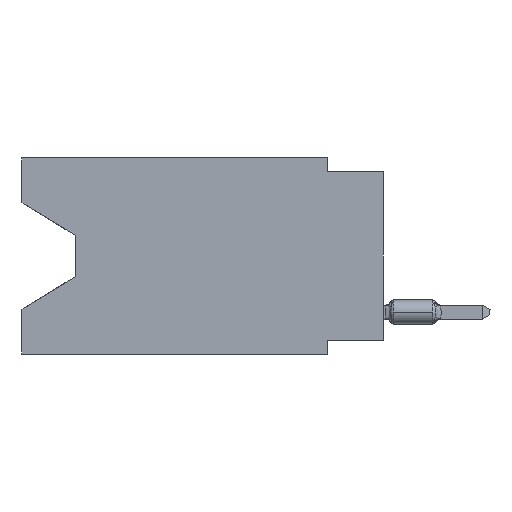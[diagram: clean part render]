
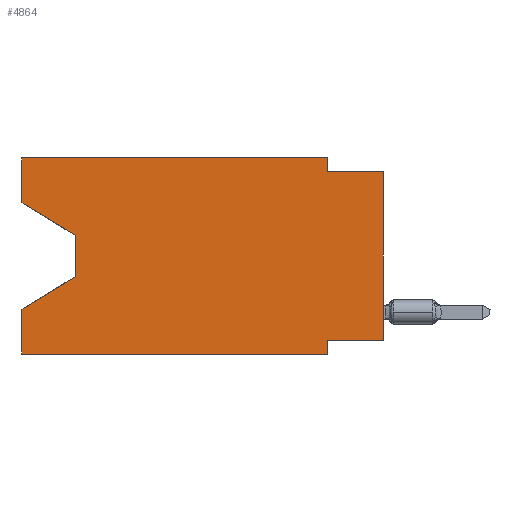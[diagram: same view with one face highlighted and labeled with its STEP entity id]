
A CAD part, left-side view. The second image highlights one B-rep face of the part: STEP entity #4864.
In plain terms, the highlighted planar face has unit normal (-1, 0, 0).
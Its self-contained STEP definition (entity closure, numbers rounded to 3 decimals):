
#112 = DIRECTION ( 'NONE',  ( 1., 0., 0. ) ) ;
#1184 = CARTESIAN_POINT ( 'NONE',  ( 0., 13.97, -5.385 ) ) ;
#3858 = VECTOR ( 'NONE', #36451, 1000. ) ;
#3903 = ORIENTED_EDGE ( 'NONE', *, *, #34705, .T. ) ;
#4229 = DIRECTION ( 'NONE',  ( 0., 1., 0. ) ) ;
#4771 = CARTESIAN_POINT ( 'NONE',  ( 0., 16.383, -6.852 ) ) ;
#4864 = ADVANCED_FACE ( 'NONE', ( #32024 ), #39775, .F. ) ;
#5009 = CARTESIAN_POINT ( 'NONE',  ( 0., 0., 0. ) ) ;
#5149 = CARTESIAN_POINT ( 'NONE',  ( 0., 2.54, 0. ) ) ;
#5249 = CARTESIAN_POINT ( 'NONE',  ( 0., 0., -8.255 ) ) ;
#6191 = DIRECTION ( 'NONE',  ( 0., 0., -1. ) ) ;
#6327 = VECTOR ( 'NONE', #29267, 1000. ) ;
#6953 = EDGE_CURVE ( 'NONE', #31298, #35868, #34721, .T. ) ;
#8057 = ORIENTED_EDGE ( 'NONE', *, *, #14320, .F. ) ;
#8295 = EDGE_CURVE ( 'NONE', #34327, #38568, #25600, .T. ) ;
#8542 = VERTEX_POINT ( 'NONE', #24056 ) ;
#9155 = EDGE_CURVE ( 'NONE', #8542, #35868, #26430, .T. ) ;
#9399 = DIRECTION ( 'NONE',  ( 0., -1., 0. ) ) ;
#9785 = DIRECTION ( 'NONE',  ( 0., 0., -1. ) ) ;
#9945 = DIRECTION ( 'NONE',  ( 0., -1., 0. ) ) ;
#10219 = ORIENTED_EDGE ( 'NONE', *, *, #41507, .T. ) ;
#10590 = CARTESIAN_POINT ( 'NONE',  ( 0., 2.54, -8.89 ) ) ;
#11214 = ORIENTED_EDGE ( 'NONE', *, *, #15917, .F. ) ;
#11377 = CARTESIAN_POINT ( 'NONE',  ( 0., 2.54, -8.255 ) ) ;
#12297 = EDGE_CURVE ( 'NONE', #21280, #42012, #35748, .T. ) ;
#12346 = VERTEX_POINT ( 'NONE', #10590 ) ;
#13457 = VERTEX_POINT ( 'NONE', #27858 ) ;
#13536 = CARTESIAN_POINT ( 'NONE',  ( 0., 0., -8.255 ) ) ;
#13543 = VERTEX_POINT ( 'NONE', #11377 ) ;
#13743 = DIRECTION ( 'NONE',  ( 0., 0.855, -0.519 ) ) ;
#14320 = EDGE_CURVE ( 'NONE', #37477, #8542, #21631, .T. ) ;
#14383 = CARTESIAN_POINT ( 'NONE',  ( 0., 13.97, -5.385 ) ) ;
#14740 = VECTOR ( 'NONE', #22101, 1000. ) ;
#14862 = EDGE_LOOP ( 'NONE', ( #21811, #34462, #3903, #35854, #10219, #37282, #26364, #19330, #38354, #8057, #11214, #35345 ) ) ;
#15600 = VECTOR ( 'NONE', #13743, 1000. ) ;
#15917 = EDGE_CURVE ( 'NONE', #13457, #37477, #33470, .T. ) ;
#16154 = CARTESIAN_POINT ( 'NONE',  ( 0., 16.383, 0. ) ) ;
#16544 = VECTOR ( 'NONE', #32602, 1000. ) ;
#16679 = CARTESIAN_POINT ( 'NONE',  ( 0., 0., -0.635 ) ) ;
#18980 = CARTESIAN_POINT ( 'NONE',  ( 0., 13.97, -3.505 ) ) ;
#18991 = VECTOR ( 'NONE', #9399, 1000. ) ;
#19330 = ORIENTED_EDGE ( 'NONE', *, *, #6953, .T. ) ;
#19361 = LINE ( 'NONE', #26292, #16544 ) ;
#19982 = CARTESIAN_POINT ( 'NONE',  ( 0., 2.54, 0. ) ) ;
#21280 = VERTEX_POINT ( 'NONE', #22576 ) ;
#21631 = LINE ( 'NONE', #5149, #28714 ) ;
#21811 = ORIENTED_EDGE ( 'NONE', *, *, #8295, .T. ) ;
#22101 = DIRECTION ( 'NONE',  ( 0., 0., 1. ) ) ;
#22576 = CARTESIAN_POINT ( 'NONE',  ( 0., 16.383, -8.89 ) ) ;
#22734 = CARTESIAN_POINT ( 'NONE',  ( 0., 16.383, 0. ) ) ;
#22752 = DIRECTION ( 'NONE',  ( 0., -0.855, -0.519 ) ) ;
#22801 = CARTESIAN_POINT ( 'NONE',  ( 0., 16.383, 0. ) ) ;
#23046 = DIRECTION ( 'NONE',  ( 0., -1., 0. ) ) ;
#23444 = LINE ( 'NONE', #22801, #3858 ) ;
#23873 = LINE ( 'NONE', #33864, #33207 ) ;
#24056 = CARTESIAN_POINT ( 'NONE',  ( 0., 2.54, -0.635 ) ) ;
#24700 = VERTEX_POINT ( 'NONE', #1184 ) ;
#24982 = EDGE_CURVE ( 'NONE', #13543, #12346, #23873, .T. ) ;
#25600 = LINE ( 'NONE', #41847, #27893 ) ;
#26109 = CARTESIAN_POINT ( 'NONE',  ( 0., 0., -0.635 ) ) ;
#26156 = DIRECTION ( 'NONE',  ( 0., 0., -1. ) ) ;
#26163 = VECTOR ( 'NONE', #9945, 1000. ) ;
#26292 = CARTESIAN_POINT ( 'NONE',  ( 0., 13.97, -3.505 ) ) ;
#26364 = ORIENTED_EDGE ( 'NONE', *, *, #27672, .F. ) ;
#26430 = LINE ( 'NONE', #16679, #26163 ) ;
#26513 = CARTESIAN_POINT ( 'NONE',  ( 0., 16.383, -8.89 ) ) ;
#27672 = EDGE_CURVE ( 'NONE', #31298, #13543, #39762, .T. ) ;
#27858 = CARTESIAN_POINT ( 'NONE',  ( 0., 16.383, 0. ) ) ;
#27893 = VECTOR ( 'NONE', #22752, 1000. ) ;
#28252 = VECTOR ( 'NONE', #4229, 1000. ) ;
#28714 = VECTOR ( 'NONE', #26156, 1000. ) ;
#29121 = EDGE_CURVE ( 'NONE', #38568, #24700, #19361, .T. ) ;
#29267 = DIRECTION ( 'NONE',  ( 0., 0., 1. ) ) ;
#30846 = VECTOR ( 'NONE', #23046, 1000. ) ;
#31298 = VERTEX_POINT ( 'NONE', #5249 ) ;
#31840 = CARTESIAN_POINT ( 'NONE',  ( 0., 16.383, -2.038 ) ) ;
#32024 = FACE_OUTER_BOUND ( 'NONE', #14862, .T. ) ;
#32602 = DIRECTION ( 'NONE',  ( 0., 0., -1. ) ) ;
#33207 = VECTOR ( 'NONE', #9785, 1000. ) ;
#33470 = LINE ( 'NONE', #36495, #18991 ) ;
#33691 = LINE ( 'NONE', #14383, #15600 ) ;
#33864 = CARTESIAN_POINT ( 'NONE',  ( 0., 2.54, -8.89 ) ) ;
#34327 = VERTEX_POINT ( 'NONE', #31840 ) ;
#34462 = ORIENTED_EDGE ( 'NONE', *, *, #29121, .T. ) ;
#34705 = EDGE_CURVE ( 'NONE', #24700, #42012, #33691, .T. ) ;
#34721 = LINE ( 'NONE', #5009, #6327 ) ;
#34949 = EDGE_CURVE ( 'NONE', #34327, #13457, #23444, .T. ) ;
#35345 = ORIENTED_EDGE ( 'NONE', *, *, #34949, .F. ) ;
#35748 = LINE ( 'NONE', #22734, #14740 ) ;
#35854 = ORIENTED_EDGE ( 'NONE', *, *, #12297, .F. ) ;
#35868 = VERTEX_POINT ( 'NONE', #26109 ) ;
#36451 = DIRECTION ( 'NONE',  ( 0., 0., 1. ) ) ;
#36495 = CARTESIAN_POINT ( 'NONE',  ( 0., 16.383, 0. ) ) ;
#37282 = ORIENTED_EDGE ( 'NONE', *, *, #24982, .F. ) ;
#37477 = VERTEX_POINT ( 'NONE', #19982 ) ;
#38354 = ORIENTED_EDGE ( 'NONE', *, *, #9155, .F. ) ;
#38568 = VERTEX_POINT ( 'NONE', #18980 ) ;
#39290 = AXIS2_PLACEMENT_3D ( 'NONE', #16154, #112, #6191 ) ;
#39762 = LINE ( 'NONE', #13536, #28252 ) ;
#39775 = PLANE ( 'NONE',  #39290 ) ;
#40388 = LINE ( 'NONE', #26513, #30846 ) ;
#41507 = EDGE_CURVE ( 'NONE', #21280, #12346, #40388, .T. ) ;
#41847 = CARTESIAN_POINT ( 'NONE',  ( 0., 16.383, -2.038 ) ) ;
#42012 = VERTEX_POINT ( 'NONE', #4771 ) ;
